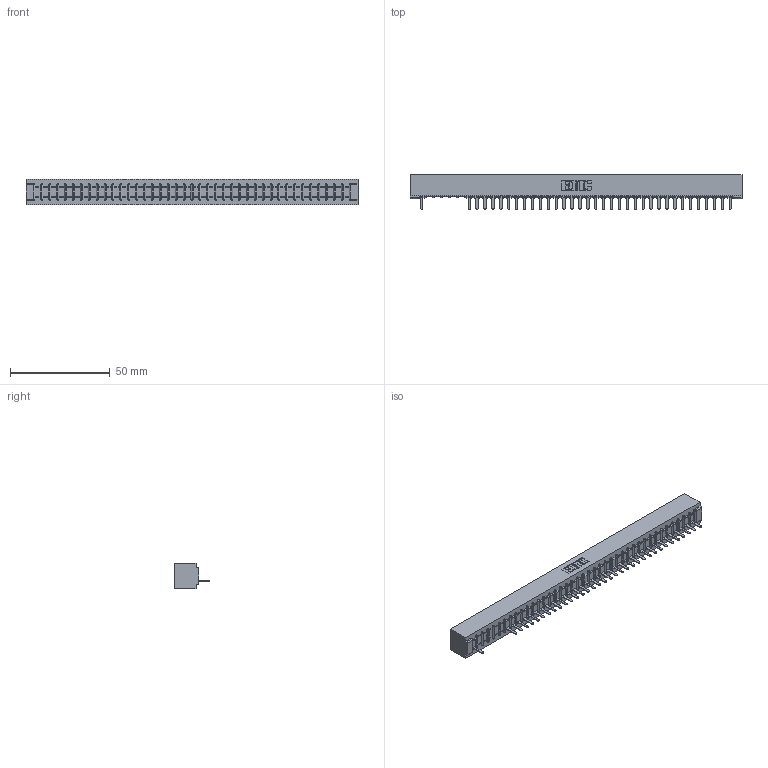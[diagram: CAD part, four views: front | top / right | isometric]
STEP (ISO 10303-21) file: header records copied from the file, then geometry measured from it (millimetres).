
FILE_DESCRIPTION (( 'STEP AP203' ), '1' );
FILE_NAME ('357-040-521-101.STEP', '2018-08-11T05:17:15', ( '' ), ( '' ), 'SwSTEP 2.0', 'SolidWorks 2016', '' );
FILE_SCHEMA (( 'CONFIG_CONTROL_DESIGN' ));
Length unit declared in the file: inch
Products named in the file (3): 307 Part_No Mounting Lugs; 307-290-002_521; 357-040-521-101
Assembly tree (36 placements, depth 2):
  357-040-521-101
    307 Part_No Mounting Lugs
    307-290-002_521  x35
Bounding box: 166.37 x 17.42 x 12.7 mm (x, y, z)
Volume: 18203.9 mm3; surface area: 22273.7 mm2
Topology: 36 solids, 36 shells, 2841 faces, 8739 edges, 5714 vertices
Faces by surface type: plane 1701, cylinder 1058, sphere 82
Entity records: 34818 total; most frequent: CARTESIAN_POINT 5895, ORIENTED_EDGE 5890, DIRECTION 5721, EDGE_CURVE 2945, LINE 2257, VECTOR 2257, VERTEX_POINT 1906, AXIS2_PLACEMENT_3D 1732
